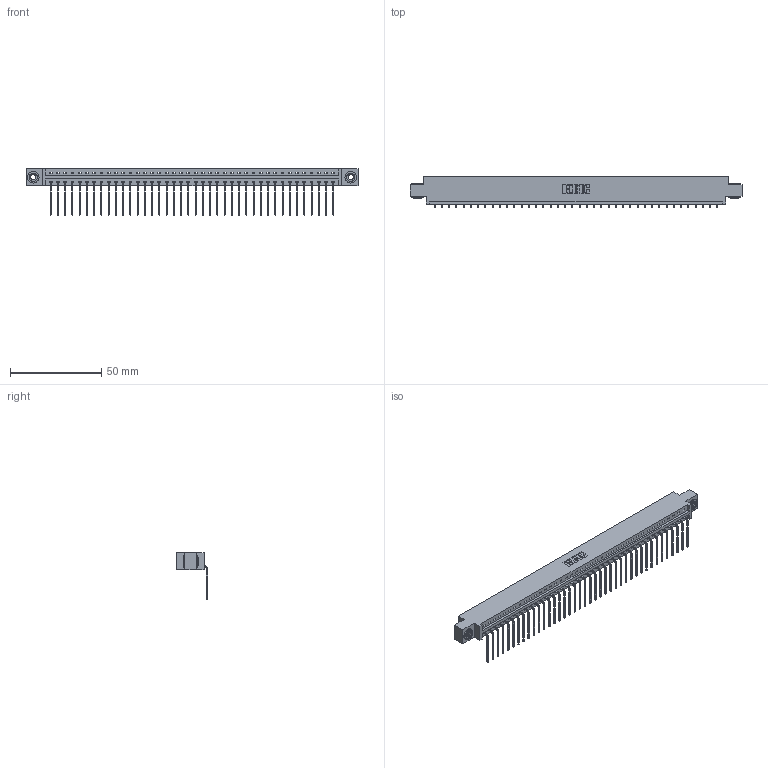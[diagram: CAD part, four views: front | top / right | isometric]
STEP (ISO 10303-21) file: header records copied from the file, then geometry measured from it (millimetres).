
FILE_DESCRIPTION (( 'STEP AP203' ), '1' );
FILE_NAME ('337-040-559-603.STEP', '2019-10-01T20:10:15', ( '' ), ( '' ), 'SwSTEP 2.0', 'SolidWorks 2016', '' );
FILE_SCHEMA (( 'CONFIG_CONTROL_DESIGN' ));
Length unit declared in the file: inch
Products named in the file (4): 337 Part_0.170 Offset - 0.156 Dia-TH; 337-040-559-603; 345-292-001_558 559 Tail - 1; 345-250-002_345-250-002-102
Assembly tree (43 placements, depth 2):
  337-040-559-603
    337 Part_0.170 Offset - 0.156 Dia-TH
    345-292-001_558 559 Tail - 1  x40
    345-250-002_345-250-002-102  x2
Bounding box: 181.51 x 17.09 x 25.53 mm (x, y, z)
Volume: 18874.9 mm3; surface area: 20641.2 mm2
Topology: 43 solids, 43 shells, 2716 faces, 8159 edges, 5382 vertices
Faces by surface type: plane 2004, cylinder 704, cone 8
Entity records: 30858 total; most frequent: CARTESIAN_POINT 5353, ORIENTED_EDGE 5322, DIRECTION 4543, EDGE_CURVE 2661, LINE 2509, VECTOR 2509, VERTEX_POINT 1770, AXIS2_PLACEMENT_3D 1017
